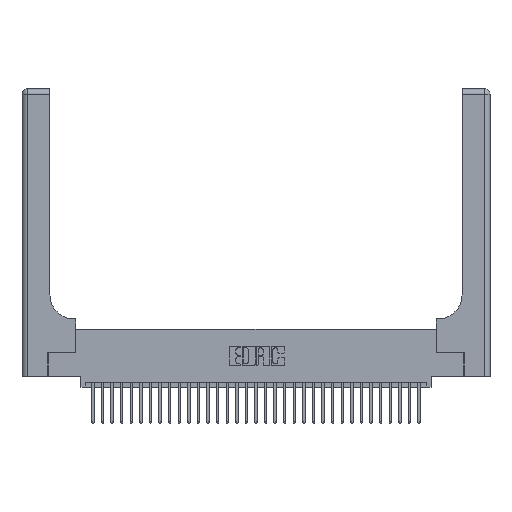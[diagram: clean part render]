
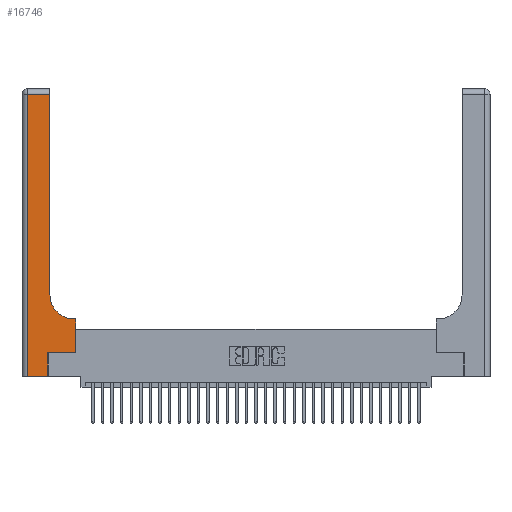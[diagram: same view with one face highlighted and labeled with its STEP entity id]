
A CAD part, top view. The second image highlights one B-rep face of the part: STEP entity #16746.
In plain terms, the highlighted planar face has unit normal (0, 0, 1).
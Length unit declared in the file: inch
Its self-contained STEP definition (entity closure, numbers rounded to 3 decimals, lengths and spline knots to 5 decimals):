
#215 = VECTOR ( 'NONE', #33064, 39.37008 ) ;
#371 = EDGE_CURVE ( 'NONE', #27642, #3809, #30856, .T. ) ;
#458 = DIRECTION ( 'NONE',  ( 0., 0., -1. ) ) ;
#661 = VERTEX_POINT ( 'NONE', #28000 ) ;
#1048 = VERTEX_POINT ( 'NONE', #30087 ) ;
#1268 = VERTEX_POINT ( 'NONE', #13952 ) ;
#1451 = FACE_OUTER_BOUND ( 'NONE', #26041, .T. ) ;
#2607 = CARTESIAN_POINT ( 'NONE',  ( 0.06, 0., 0.37 ) ) ;
#2757 = VERTEX_POINT ( 'NONE', #16133 ) ;
#2909 = EDGE_CURVE ( 'NONE', #10045, #2757, #21752, .T. ) ;
#2937 = DIRECTION ( 'NONE',  ( 0., -1., 0. ) ) ;
#3278 = CARTESIAN_POINT ( 'NONE',  ( 0.06, 3., 0.37 ) ) ;
#3356 = CARTESIAN_POINT ( 'NONE',  ( 0., 0., 0.37 ) ) ;
#3809 = VERTEX_POINT ( 'NONE', #6330 ) ;
#5048 = VERTEX_POINT ( 'NONE', #19920 ) ;
#5477 = DIRECTION ( 'NONE',  ( -1., 0., 0. ) ) ;
#5510 = EDGE_CURVE ( 'NONE', #1268, #5048, #28545, .T. ) ;
#6330 = CARTESIAN_POINT ( 'NONE',  ( 0.269, 0., 0.37 ) ) ;
#6922 = VECTOR ( 'NONE', #5477, 39.37008 ) ;
#7393 = LINE ( 'NONE', #3278, #23747 ) ;
#7403 = LINE ( 'NONE', #24175, #22519 ) ;
#7735 = ORIENTED_EDGE ( 'NONE', *, *, #26723, .T. ) ;
#8952 = EDGE_CURVE ( 'NONE', #24016, #661, #31132, .T. ) ;
#9520 = VECTOR ( 'NONE', #18070, 39.37008 ) ;
#9563 = LINE ( 'NONE', #24094, #20187 ) ;
#9808 = EDGE_CURVE ( 'NONE', #5048, #27642, #7393, .T. ) ;
#10045 = VERTEX_POINT ( 'NONE', #27925 ) ;
#10249 = CARTESIAN_POINT ( 'NONE',  ( 0., 3., 0.37 ) ) ;
#12259 = ORIENTED_EDGE ( 'NONE', *, *, #16785, .T. ) ;
#12388 = ORIENTED_EDGE ( 'NONE', *, *, #371, .T. ) ;
#12620 = CARTESIAN_POINT ( 'NONE',  ( 0.269, 0.25, 0.37 ) ) ;
#12905 = DIRECTION ( 'NONE',  ( 0., 0., -1. ) ) ;
#12987 = ORIENTED_EDGE ( 'NONE', *, *, #2909, .T. ) ;
#13449 = CARTESIAN_POINT ( 'NONE',  ( 0.5415, 0.85, 0.37 ) ) ;
#13952 = CARTESIAN_POINT ( 'NONE',  ( 0.2915, 2.94, 0.37 ) ) ;
#14725 = CARTESIAN_POINT ( 'NONE',  ( 0.2915, 3., 0.37 ) ) ;
#15526 = EDGE_CURVE ( 'NONE', #2757, #1268, #27597, .T. ) ;
#16133 = CARTESIAN_POINT ( 'NONE',  ( 0.2915, 0.85, 0.37 ) ) ;
#16746 = ADVANCED_FACE ( 'NONE', ( #1451 ), #31461, .F. ) ;
#16785 = EDGE_CURVE ( 'NONE', #1048, #10045, #9563, .T. ) ;
#16909 = ORIENTED_EDGE ( 'NONE', *, *, #9808, .T. ) ;
#18070 = DIRECTION ( 'NONE',  ( 1., 0., 0. ) ) ;
#18287 = AXIS2_PLACEMENT_3D ( 'NONE', #10249, #12905, #31122 ) ;
#18307 = ORIENTED_EDGE ( 'NONE', *, *, #5510, .T. ) ;
#18723 = DIRECTION ( 'NONE',  ( -1., 0., 0. ) ) ;
#19920 = CARTESIAN_POINT ( 'NONE',  ( 0.06, 2.94, 0.37 ) ) ;
#20187 = VECTOR ( 'NONE', #18723, 39.37008 ) ;
#20337 = CARTESIAN_POINT ( 'NONE',  ( 0., 2.94, 0.37 ) ) ;
#21333 = DIRECTION ( 'NONE',  ( 1., 0., 0. ) ) ;
#21641 = DIRECTION ( 'NONE',  ( 1., 0., 0. ) ) ;
#21752 = CIRCLE ( 'NONE', #24744, 0.25 ) ;
#22519 = VECTOR ( 'NONE', #31783, 39.37008 ) ;
#23747 = VECTOR ( 'NONE', #2937, 39.37008 ) ;
#24016 = VERTEX_POINT ( 'NONE', #26594 ) ;
#24094 = CARTESIAN_POINT ( 'NONE',  ( 0.2915, 0.6, 0.37 ) ) ;
#24175 = CARTESIAN_POINT ( 'NONE',  ( 0.269, 0., 0.37 ) ) ;
#24483 = ORIENTED_EDGE ( 'NONE', *, *, #8952, .T. ) ;
#24744 = AXIS2_PLACEMENT_3D ( 'NONE', #13449, #458, #21333 ) ;
#26041 = EDGE_LOOP ( 'NONE', ( #26147, #18307, #16909, #12388, #26936, #24483, #7735, #12259, #12987 ) ) ;
#26147 = ORIENTED_EDGE ( 'NONE', *, *, #15526, .T. ) ;
#26394 = VECTOR ( 'NONE', #21641, 39.37008 ) ;
#26594 = CARTESIAN_POINT ( 'NONE',  ( 0.269, 0.25, 0.37 ) ) ;
#26723 = EDGE_CURVE ( 'NONE', #661, #1048, #29813, .T. ) ;
#26936 = ORIENTED_EDGE ( 'NONE', *, *, #29727, .T. ) ;
#27597 = LINE ( 'NONE', #14725, #215 ) ;
#27642 = VERTEX_POINT ( 'NONE', #2607 ) ;
#27925 = CARTESIAN_POINT ( 'NONE',  ( 0.5415, 0.6, 0.37 ) ) ;
#28000 = CARTESIAN_POINT ( 'NONE',  ( 0.5585, 0.25, 0.37 ) ) ;
#28545 = LINE ( 'NONE', #20337, #6922 ) ;
#28581 = VECTOR ( 'NONE', #28910, 39.37008 ) ;
#28910 = DIRECTION ( 'NONE',  ( 0., 1., 0. ) ) ;
#29727 = EDGE_CURVE ( 'NONE', #3809, #24016, #7403, .T. ) ;
#29813 = LINE ( 'NONE', #31648, #28581 ) ;
#30087 = CARTESIAN_POINT ( 'NONE',  ( 0.5585, 0.6, 0.37 ) ) ;
#30856 = LINE ( 'NONE', #3356, #26394 ) ;
#31122 = DIRECTION ( 'NONE',  ( -1., 0., 0. ) ) ;
#31132 = LINE ( 'NONE', #12620, #9520 ) ;
#31461 = PLANE ( 'NONE',  #18287 ) ;
#31648 = CARTESIAN_POINT ( 'NONE',  ( 0.5585, 0.25, 0.37 ) ) ;
#31783 = DIRECTION ( 'NONE',  ( 0., 1., 0. ) ) ;
#33064 = DIRECTION ( 'NONE',  ( 0., 1., 0. ) ) ;
